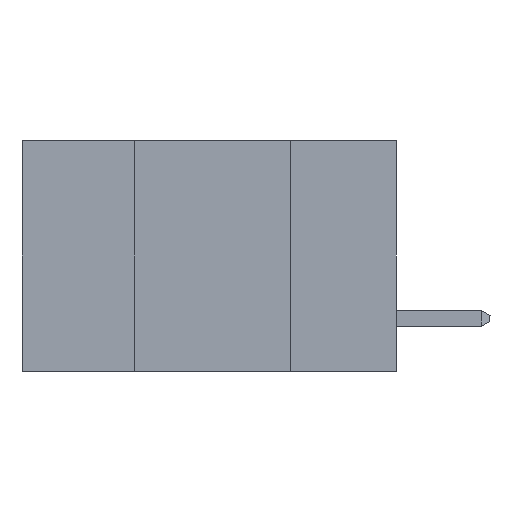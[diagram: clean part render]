
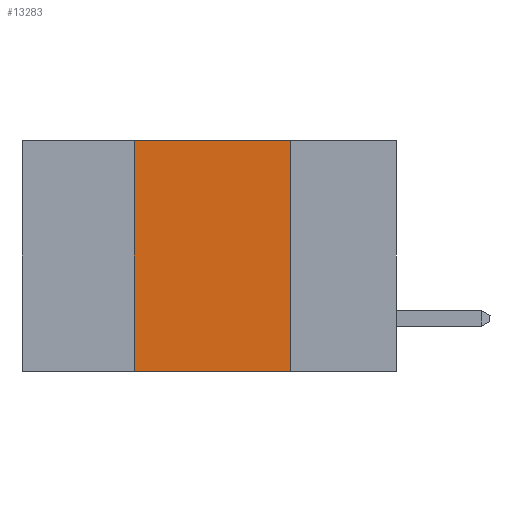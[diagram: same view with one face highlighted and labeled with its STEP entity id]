
A CAD part, left-side view. The second image highlights one B-rep face of the part: STEP entity #13283.
In plain terms, the highlighted planar face has unit normal (-1, 0, 0).
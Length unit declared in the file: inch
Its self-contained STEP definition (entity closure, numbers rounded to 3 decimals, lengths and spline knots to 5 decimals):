
#887 = VECTOR ( 'NONE', #2449, 39.37008 ) ;
#1004 = CARTESIAN_POINT ( 'NONE',  ( 0., 0.17, -0.37 ) ) ;
#1613 = LINE ( 'NONE', #10610, #4228 ) ;
#2449 = DIRECTION ( 'NONE',  ( 0., -1., 0. ) ) ;
#2860 = CARTESIAN_POINT ( 'NONE',  ( 0., 0.17, 0. ) ) ;
#3289 = DIRECTION ( 'NONE',  ( 1., 0., 0. ) ) ;
#3506 = PLANE ( 'NONE',  #9231 ) ;
#3827 = EDGE_CURVE ( 'NONE', #13412, #9416, #20447, .T. ) ;
#4228 = VECTOR ( 'NONE', #8922, 39.37008 ) ;
#4354 = LINE ( 'NONE', #9625, #887 ) ;
#5149 = ORIENTED_EDGE ( 'NONE', *, *, #18487, .T. ) ;
#7120 = CARTESIAN_POINT ( 'NONE',  ( 0., 0.42, -0.37 ) ) ;
#7570 = ORIENTED_EDGE ( 'NONE', *, *, #3827, .F. ) ;
#8130 = CARTESIAN_POINT ( 'NONE',  ( 0., 0.42, -0.37 ) ) ;
#8533 = CARTESIAN_POINT ( 'NONE',  ( 0., 0.6, 0. ) ) ;
#8580 = VECTOR ( 'NONE', #15540, 39.37008 ) ;
#8922 = DIRECTION ( 'NONE',  ( 0., 0., -1. ) ) ;
#9231 = AXIS2_PLACEMENT_3D ( 'NONE', #10373, #3289, #20610 ) ;
#9416 = VERTEX_POINT ( 'NONE', #2860 ) ;
#9625 = CARTESIAN_POINT ( 'NONE',  ( 0., 0.6, -0.37 ) ) ;
#10152 = FACE_OUTER_BOUND ( 'NONE', #14977, .T. ) ;
#10373 = CARTESIAN_POINT ( 'NONE',  ( 0., 0.6, 0. ) ) ;
#10610 = CARTESIAN_POINT ( 'NONE',  ( 0., 0.17, -0.37 ) ) ;
#11249 = EDGE_CURVE ( 'NONE', #12417, #13412, #15647, .T. ) ;
#12015 = DIRECTION ( 'NONE',  ( 0., -1., 0. ) ) ;
#12417 = VERTEX_POINT ( 'NONE', #8130 ) ;
#12901 = ORIENTED_EDGE ( 'NONE', *, *, #14527, .F. ) ;
#13283 = ADVANCED_FACE ( 'NONE', ( #10152 ), #3506, .F. ) ;
#13412 = VERTEX_POINT ( 'NONE', #14307 ) ;
#14307 = CARTESIAN_POINT ( 'NONE',  ( 0., 0.42, 0. ) ) ;
#14527 = EDGE_CURVE ( 'NONE', #9416, #21293, #1613, .T. ) ;
#14803 = VECTOR ( 'NONE', #12015, 39.37008 ) ;
#14977 = EDGE_LOOP ( 'NONE', ( #12901, #7570, #21728, #5149 ) ) ;
#15540 = DIRECTION ( 'NONE',  ( 0., 0., 1. ) ) ;
#15647 = LINE ( 'NONE', #7120, #8580 ) ;
#18487 = EDGE_CURVE ( 'NONE', #12417, #21293, #4354, .T. ) ;
#20447 = LINE ( 'NONE', #8533, #14803 ) ;
#20610 = DIRECTION ( 'NONE',  ( 0., 0., -1. ) ) ;
#21293 = VERTEX_POINT ( 'NONE', #1004 ) ;
#21728 = ORIENTED_EDGE ( 'NONE', *, *, #11249, .F. ) ;
